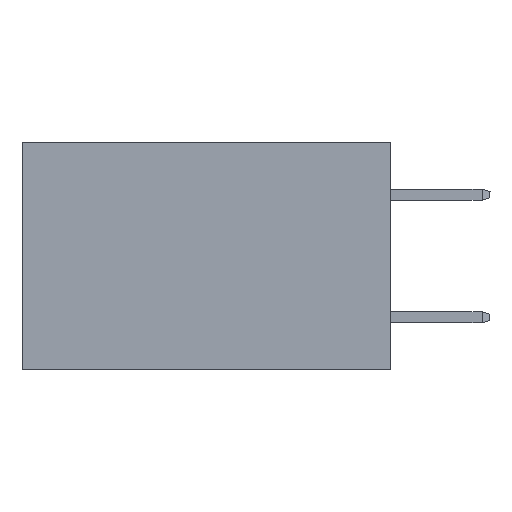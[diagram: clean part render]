
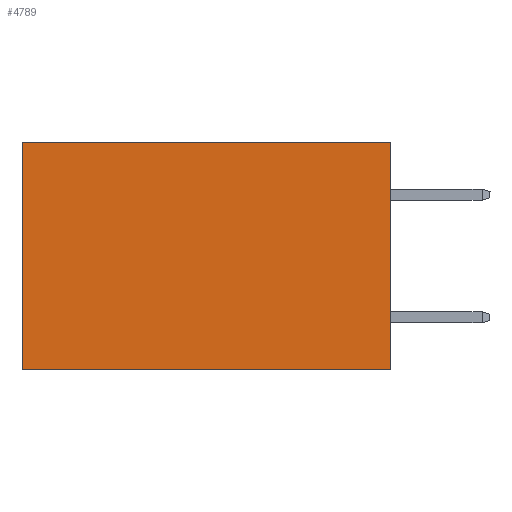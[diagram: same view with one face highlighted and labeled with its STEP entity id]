
A CAD part, left-side view. The second image highlights one B-rep face of the part: STEP entity #4789.
In plain terms, the highlighted planar face has unit normal (-1, 0, 0).
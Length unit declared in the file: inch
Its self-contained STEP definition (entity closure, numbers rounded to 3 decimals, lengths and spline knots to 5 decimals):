
#48 = EDGE_LOOP ( 'NONE', ( #11376, #10573, #14865, #2641 ) ) ;
#119 = FACE_OUTER_BOUND ( 'NONE', #48, .T. ) ;
#889 = EDGE_CURVE ( 'NONE', #3761, #5579, #2918, .T. ) ;
#1075 = LINE ( 'NONE', #6402, #8000 ) ;
#1085 = DIRECTION ( 'NONE',  ( 0., 0., -1. ) ) ;
#1953 = LINE ( 'NONE', #10482, #14000 ) ;
#2641 = ORIENTED_EDGE ( 'NONE', *, *, #8409, .T. ) ;
#2726 = VERTEX_POINT ( 'NONE', #5729 ) ;
#2918 = LINE ( 'NONE', #15448, #5382 ) ;
#3086 = VECTOR ( 'NONE', #7162, 39.37008 ) ;
#3761 = VERTEX_POINT ( 'NONE', #8503 ) ;
#3805 = CARTESIAN_POINT ( 'NONE',  ( 0.2875, 0., 0. ) ) ;
#4789 = ADVANCED_FACE ( 'NONE', ( #119 ), #5443, .F. ) ;
#4862 = DIRECTION ( 'NONE',  ( 0., 1., 0. ) ) ;
#5382 = VECTOR ( 'NONE', #7168, 39.37008 ) ;
#5443 = PLANE ( 'NONE',  #7509 ) ;
#5579 = VERTEX_POINT ( 'NONE', #9876 ) ;
#5729 = CARTESIAN_POINT ( 'NONE',  ( 0.2875, 0., -0.37 ) ) ;
#6402 = CARTESIAN_POINT ( 'NONE',  ( 0.2875, 0., 0. ) ) ;
#7022 = VERTEX_POINT ( 'NONE', #3805 ) ;
#7159 = EDGE_CURVE ( 'NONE', #2726, #5579, #1953, .T. ) ;
#7162 = DIRECTION ( 'NONE',  ( 0., 0., -1. ) ) ;
#7168 = DIRECTION ( 'NONE',  ( 0., 0., -1. ) ) ;
#7509 = AXIS2_PLACEMENT_3D ( 'NONE', #15422, #18110, #1085 ) ;
#8000 = VECTOR ( 'NONE', #4862, 39.37008 ) ;
#8409 = EDGE_CURVE ( 'NONE', #7022, #3761, #1075, .T. ) ;
#8503 = CARTESIAN_POINT ( 'NONE',  ( 0.2875, 0.6, 0. ) ) ;
#8654 = CARTESIAN_POINT ( 'NONE',  ( 0.2875, 0., 0. ) ) ;
#8680 = LINE ( 'NONE', #8654, #3086 ) ;
#9876 = CARTESIAN_POINT ( 'NONE',  ( 0.2875, 0.6, -0.37 ) ) ;
#10482 = CARTESIAN_POINT ( 'NONE',  ( 0.2875, 0., -0.37 ) ) ;
#10540 = DIRECTION ( 'NONE',  ( 0., 1., 0. ) ) ;
#10573 = ORIENTED_EDGE ( 'NONE', *, *, #7159, .F. ) ;
#11376 = ORIENTED_EDGE ( 'NONE', *, *, #889, .T. ) ;
#14000 = VECTOR ( 'NONE', #10540, 39.37008 ) ;
#14865 = ORIENTED_EDGE ( 'NONE', *, *, #18256, .F. ) ;
#15422 = CARTESIAN_POINT ( 'NONE',  ( 0.2875, 0., 0. ) ) ;
#15448 = CARTESIAN_POINT ( 'NONE',  ( 0.2875, 0.6, 0. ) ) ;
#18110 = DIRECTION ( 'NONE',  ( 1., 0., 0. ) ) ;
#18256 = EDGE_CURVE ( 'NONE', #7022, #2726, #8680, .T. ) ;
